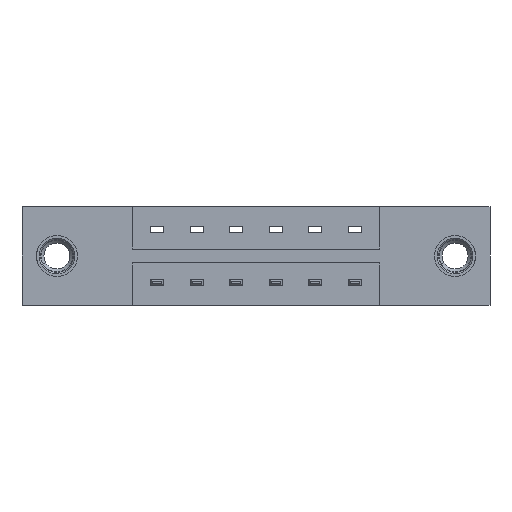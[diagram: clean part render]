
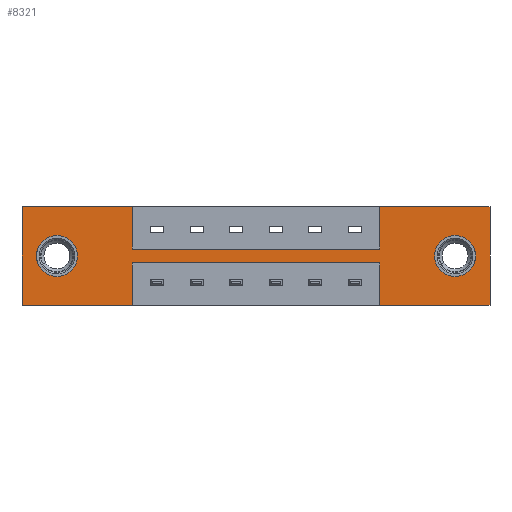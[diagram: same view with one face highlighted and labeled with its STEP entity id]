
A CAD part, front view. The second image highlights one B-rep face of the part: STEP entity #8321.
In plain terms, the highlighted planar face has unit normal (0, -1, 0).
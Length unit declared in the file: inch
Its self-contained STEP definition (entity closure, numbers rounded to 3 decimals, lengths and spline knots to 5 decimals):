
#17 = LINE ( 'NONE', #697, #7134 ) ;
#29 = CARTESIAN_POINT ( 'NONE',  ( 1.6425, 0., -0.1875 ) ) ;
#75 = ORIENTED_EDGE ( 'NONE', *, *, #6229, .F. ) ;
#81 = ORIENTED_EDGE ( 'NONE', *, *, #1880, .F. ) ;
#269 = DIRECTION ( 'NONE',  ( -1., 0., 0. ) ) ;
#297 = LINE ( 'NONE', #1809, #619 ) ;
#303 = VECTOR ( 'NONE', #443, 39.37008 ) ;
#356 = CARTESIAN_POINT ( 'NONE',  ( 1.6425, 0., -0.1875 ) ) ;
#421 = DIRECTION ( 'NONE',  ( 0., 1., 0. ) ) ;
#438 = CARTESIAN_POINT ( 'NONE',  ( 0.4175, 0., -0.375 ) ) ;
#443 = DIRECTION ( 'NONE',  ( 1., 0., 0. ) ) ;
#465 = CARTESIAN_POINT ( 'NONE',  ( 1.3575, 0., -0.161 ) ) ;
#532 = CARTESIAN_POINT ( 'NONE',  ( 0., 0., 0. ) ) ;
#587 = EDGE_CURVE ( 'NONE', #9031, #6523, #2776, .T. ) ;
#593 = VERTEX_POINT ( 'NONE', #4519 ) ;
#594 = FACE_BOUND ( 'NONE', #6867, .T. ) ;
#619 = VECTOR ( 'NONE', #269, 39.37008 ) ;
#687 = CARTESIAN_POINT ( 'NONE',  ( 1.3575, 0., -0.375 ) ) ;
#697 = CARTESIAN_POINT ( 'NONE',  ( 0., 0., 0. ) ) ;
#830 = CARTESIAN_POINT ( 'NONE',  ( 1.3575, 0., 0. ) ) ;
#855 = VECTOR ( 'NONE', #1495, 39.37008 ) ;
#904 = CARTESIAN_POINT ( 'NONE',  ( 1.6425, 0., -0.2655 ) ) ;
#947 = VERTEX_POINT ( 'NONE', #465 ) ;
#957 = DIRECTION ( 'NONE',  ( 1., 0., 0. ) ) ;
#967 = DIRECTION ( 'NONE',  ( 0., 1., 0. ) ) ;
#983 = CARTESIAN_POINT ( 'NONE',  ( 0.4175, 0., 0. ) ) ;
#1069 = CARTESIAN_POINT ( 'NONE',  ( 1.775, 0., 0. ) ) ;
#1079 = VECTOR ( 'NONE', #2364, 39.37008 ) ;
#1112 = VERTEX_POINT ( 'NONE', #687 ) ;
#1129 = DIRECTION ( 'NONE',  ( 0., 0., -1. ) ) ;
#1293 = LINE ( 'NONE', #5185, #1079 ) ;
#1495 = DIRECTION ( 'NONE',  ( -1., 0., 0. ) ) ;
#1616 = CARTESIAN_POINT ( 'NONE',  ( 0.4175, 0., -0.214 ) ) ;
#1650 = LINE ( 'NONE', #2169, #855 ) ;
#1809 = CARTESIAN_POINT ( 'NONE',  ( 0., 0., -0.375 ) ) ;
#1813 = DIRECTION ( 'NONE',  ( 0., 1., 0. ) ) ;
#1827 = EDGE_CURVE ( 'NONE', #9185, #1112, #1650, .T. ) ;
#1880 = EDGE_CURVE ( 'NONE', #947, #4030, #1293, .T. ) ;
#2001 = DIRECTION ( 'NONE',  ( 0., 0., 1. ) ) ;
#2126 = EDGE_CURVE ( 'NONE', #593, #5137, #4220, .T. ) ;
#2169 = CARTESIAN_POINT ( 'NONE',  ( 0., 0., -0.375 ) ) ;
#2207 = EDGE_CURVE ( 'NONE', #2348, #9184, #6040, .T. ) ;
#2220 = ORIENTED_EDGE ( 'NONE', *, *, #7577, .F. ) ;
#2294 = CARTESIAN_POINT ( 'NONE',  ( 1.3575, 0., -0.214 ) ) ;
#2303 = ORIENTED_EDGE ( 'NONE', *, *, #5729, .T. ) ;
#2348 = VERTEX_POINT ( 'NONE', #7191 ) ;
#2364 = DIRECTION ( 'NONE',  ( 0., 0., 1. ) ) ;
#2368 = DIRECTION ( 'NONE',  ( 0., 0., 1. ) ) ;
#2497 = EDGE_CURVE ( 'NONE', #4030, #4258, #17, .T. ) ;
#2545 = AXIS2_PLACEMENT_3D ( 'NONE', #29, #8735, #6601 ) ;
#2592 = ORIENTED_EDGE ( 'NONE', *, *, #3610, .F. ) ;
#2623 = LINE ( 'NONE', #2294, #5554 ) ;
#2641 = ORIENTED_EDGE ( 'NONE', *, *, #3950, .T. ) ;
#2776 = CIRCLE ( 'NONE', #4699, 0.078 ) ;
#2838 = VECTOR ( 'NONE', #2001, 39.37008 ) ;
#2840 = EDGE_LOOP ( 'NONE', ( #75, #3621, #2592, #7901, #81, #2220, #7597, #5861, #4708, #7574, #8238, #8964 ) ) ;
#2952 = CARTESIAN_POINT ( 'NONE',  ( 0.4175, 0., -0.161 ) ) ;
#2955 = VERTEX_POINT ( 'NONE', #4939 ) ;
#2994 = VECTOR ( 'NONE', #5421, 39.37008 ) ;
#3130 = CARTESIAN_POINT ( 'NONE',  ( 0.1325, 0., -0.1875 ) ) ;
#3317 = CARTESIAN_POINT ( 'NONE',  ( 0.1325, 0., -0.1095 ) ) ;
#3414 = EDGE_CURVE ( 'NONE', #4303, #4374, #297, .T. ) ;
#3430 = CIRCLE ( 'NONE', #2545, 0.078 ) ;
#3450 = CARTESIAN_POINT ( 'NONE',  ( 0.4175, 0., -0.161 ) ) ;
#3465 = CARTESIAN_POINT ( 'NONE',  ( 0., 0., -0.375 ) ) ;
#3574 = CARTESIAN_POINT ( 'NONE',  ( 0.1325, 0., -0.2655 ) ) ;
#3610 = EDGE_CURVE ( 'NONE', #4258, #9185, #4903, .T. ) ;
#3621 = ORIENTED_EDGE ( 'NONE', *, *, #1827, .F. ) ;
#3892 = CARTESIAN_POINT ( 'NONE',  ( 0.4175, 0., -0.214 ) ) ;
#3950 = EDGE_CURVE ( 'NONE', #5137, #593, #3430, .T. ) ;
#4030 = VERTEX_POINT ( 'NONE', #830 ) ;
#4071 = CARTESIAN_POINT ( 'NONE',  ( 0.4175, 0., -0.214 ) ) ;
#4090 = DIRECTION ( 'NONE',  ( 0., -1., 0. ) ) ;
#4220 = CIRCLE ( 'NONE', #5711, 0.078 ) ;
#4244 = EDGE_LOOP ( 'NONE', ( #2303, #5622 ) ) ;
#4258 = VERTEX_POINT ( 'NONE', #6124 ) ;
#4303 = VERTEX_POINT ( 'NONE', #438 ) ;
#4327 = LINE ( 'NONE', #7885, #6821 ) ;
#4374 = VERTEX_POINT ( 'NONE', #3465 ) ;
#4440 = FACE_OUTER_BOUND ( 'NONE', #2840, .T. ) ;
#4519 = CARTESIAN_POINT ( 'NONE',  ( 1.6425, 0., -0.1095 ) ) ;
#4545 = EDGE_CURVE ( 'NONE', #8730, #8999, #4327, .T. ) ;
#4549 = DIRECTION ( 'NONE',  ( 0., 0., 1. ) ) ;
#4699 = AXIS2_PLACEMENT_3D ( 'NONE', #8826, #967, #4549 ) ;
#4708 = ORIENTED_EDGE ( 'NONE', *, *, #6093, .F. ) ;
#4802 = CARTESIAN_POINT ( 'NONE',  ( 0., 0., 0. ) ) ;
#4903 = LINE ( 'NONE', #1069, #2994 ) ;
#4939 = CARTESIAN_POINT ( 'NONE',  ( 0., 0., 0. ) ) ;
#5033 = ORIENTED_EDGE ( 'NONE', *, *, #2126, .T. ) ;
#5137 = VERTEX_POINT ( 'NONE', #904 ) ;
#5185 = CARTESIAN_POINT ( 'NONE',  ( 1.3575, 0., -0.161 ) ) ;
#5202 = DIRECTION ( 'NONE',  ( 0., 0., -1. ) ) ;
#5216 = VECTOR ( 'NONE', #5202, 39.37008 ) ;
#5220 = FACE_BOUND ( 'NONE', #4244, .T. ) ;
#5305 = DIRECTION ( 'NONE',  ( 0., 0., 1. ) ) ;
#5358 = VECTOR ( 'NONE', #7093, 39.37008 ) ;
#5421 = DIRECTION ( 'NONE',  ( 0., 0., -1. ) ) ;
#5554 = VECTOR ( 'NONE', #2368, 39.37008 ) ;
#5622 = ORIENTED_EDGE ( 'NONE', *, *, #587, .T. ) ;
#5670 = EDGE_CURVE ( 'NONE', #9184, #4303, #7129, .T. ) ;
#5711 = AXIS2_PLACEMENT_3D ( 'NONE', #356, #421, #1129 ) ;
#5729 = EDGE_CURVE ( 'NONE', #6523, #9031, #5906, .T. ) ;
#5769 = AXIS2_PLACEMENT_3D ( 'NONE', #8416, #4090, #9116 ) ;
#5807 = LINE ( 'NONE', #2952, #7390 ) ;
#5861 = ORIENTED_EDGE ( 'NONE', *, *, #9269, .F. ) ;
#5906 = CIRCLE ( 'NONE', #6297, 0.078 ) ;
#6040 = LINE ( 'NONE', #4071, #5358 ) ;
#6093 = EDGE_CURVE ( 'NONE', #4374, #2955, #7227, .T. ) ;
#6124 = CARTESIAN_POINT ( 'NONE',  ( 1.775, 0., 0. ) ) ;
#6229 = EDGE_CURVE ( 'NONE', #1112, #2348, #2623, .T. ) ;
#6297 = AXIS2_PLACEMENT_3D ( 'NONE', #3130, #1813, #5305 ) ;
#6474 = DIRECTION ( 'NONE',  ( 1., 0., 0. ) ) ;
#6523 = VERTEX_POINT ( 'NONE', #3317 ) ;
#6601 = DIRECTION ( 'NONE',  ( 0., 0., -1. ) ) ;
#6821 = VECTOR ( 'NONE', #8630, 39.37008 ) ;
#6867 = EDGE_LOOP ( 'NONE', ( #5033, #2641 ) ) ;
#7093 = DIRECTION ( 'NONE',  ( -1., 0., 0. ) ) ;
#7129 = LINE ( 'NONE', #1616, #5216 ) ;
#7134 = VECTOR ( 'NONE', #6474, 39.37008 ) ;
#7191 = CARTESIAN_POINT ( 'NONE',  ( 1.3575, 0., -0.214 ) ) ;
#7227 = LINE ( 'NONE', #532, #2838 ) ;
#7390 = VECTOR ( 'NONE', #957, 39.37008 ) ;
#7574 = ORIENTED_EDGE ( 'NONE', *, *, #3414, .F. ) ;
#7577 = EDGE_CURVE ( 'NONE', #8999, #947, #5807, .T. ) ;
#7597 = ORIENTED_EDGE ( 'NONE', *, *, #4545, .F. ) ;
#7885 = CARTESIAN_POINT ( 'NONE',  ( 0.4175, 0., -0.161 ) ) ;
#7901 = ORIENTED_EDGE ( 'NONE', *, *, #2497, .F. ) ;
#8193 = CARTESIAN_POINT ( 'NONE',  ( 1.775, 0., -0.375 ) ) ;
#8238 = ORIENTED_EDGE ( 'NONE', *, *, #5670, .F. ) ;
#8321 = ADVANCED_FACE ( 'NONE', ( #594, #5220, #4440 ), #8383, .T. ) ;
#8383 = PLANE ( 'NONE',  #5769 ) ;
#8416 = CARTESIAN_POINT ( 'NONE',  ( 0., 0., -0.375 ) ) ;
#8520 = LINE ( 'NONE', #4802, #303 ) ;
#8630 = DIRECTION ( 'NONE',  ( 0., 0., -1. ) ) ;
#8730 = VERTEX_POINT ( 'NONE', #983 ) ;
#8735 = DIRECTION ( 'NONE',  ( 0., 1., 0. ) ) ;
#8826 = CARTESIAN_POINT ( 'NONE',  ( 0.1325, 0., -0.1875 ) ) ;
#8964 = ORIENTED_EDGE ( 'NONE', *, *, #2207, .F. ) ;
#8999 = VERTEX_POINT ( 'NONE', #3450 ) ;
#9031 = VERTEX_POINT ( 'NONE', #3574 ) ;
#9116 = DIRECTION ( 'NONE',  ( 0., 0., -1. ) ) ;
#9184 = VERTEX_POINT ( 'NONE', #3892 ) ;
#9185 = VERTEX_POINT ( 'NONE', #8193 ) ;
#9269 = EDGE_CURVE ( 'NONE', #2955, #8730, #8520, .T. ) ;
